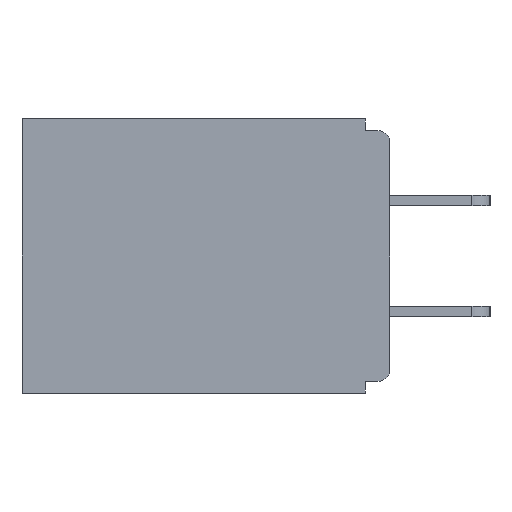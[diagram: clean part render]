
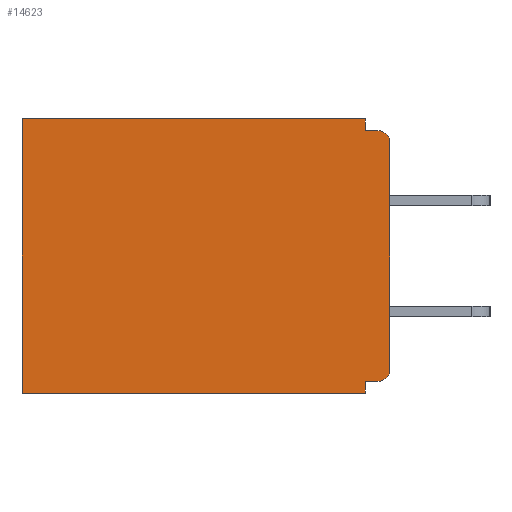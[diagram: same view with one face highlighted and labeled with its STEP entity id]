
A CAD part, left-side view. The second image highlights one B-rep face of the part: STEP entity #14623.
In plain terms, the highlighted planar face has unit normal (-1, 0, 0).
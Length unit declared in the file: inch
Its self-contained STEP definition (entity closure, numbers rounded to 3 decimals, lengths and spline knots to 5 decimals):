
#581 = CARTESIAN_POINT ( 'NONE',  ( 0.298, 0., -0.03 ) ) ;
#639 = CARTESIAN_POINT ( 'NONE',  ( 0.298, 0.46, 0. ) ) ;
#872 = VERTEX_POINT ( 'NONE', #6271 ) ;
#1793 = EDGE_CURVE ( 'NONE', #19414, #14546, #3138, .T. ) ;
#1974 = ORIENTED_EDGE ( 'NONE', *, *, #3672, .F. ) ;
#2142 = EDGE_CURVE ( 'NONE', #9829, #6226, #15710, .T. ) ;
#2200 = EDGE_CURVE ( 'NONE', #872, #7360, #11636, .T. ) ;
#2210 = CARTESIAN_POINT ( 'NONE',  ( 0.298, 0.46, -0.343 ) ) ;
#2600 = CARTESIAN_POINT ( 'NONE',  ( 0.298, 0.031, -0.343 ) ) ;
#2861 = CARTESIAN_POINT ( 'NONE',  ( 0.298, 0.015, -0.015 ) ) ;
#3009 = EDGE_CURVE ( 'NONE', #4221, #872, #5028, .T. ) ;
#3138 = LINE ( 'NONE', #11906, #14774 ) ;
#3296 = CARTESIAN_POINT ( 'NONE',  ( 0.298, 0.015, -0.328 ) ) ;
#3672 = EDGE_CURVE ( 'NONE', #4221, #16984, #13255, .T. ) ;
#4221 = VERTEX_POINT ( 'NONE', #19803 ) ;
#4634 = FACE_OUTER_BOUND ( 'NONE', #7765, .T. ) ;
#4674 = DIRECTION ( 'NONE',  ( -1., 0., 0. ) ) ;
#5028 = LINE ( 'NONE', #6264, #16907 ) ;
#5146 = CARTESIAN_POINT ( 'NONE',  ( 0.298, 0., -0.015 ) ) ;
#5211 = DIRECTION ( 'NONE',  ( 0., 0., -1. ) ) ;
#5227 = ORIENTED_EDGE ( 'NONE', *, *, #12411, .F. ) ;
#6051 = PLANE ( 'NONE',  #15280 ) ;
#6153 = VECTOR ( 'NONE', #16718, 39.37008 ) ;
#6226 = VERTEX_POINT ( 'NONE', #2861 ) ;
#6264 = CARTESIAN_POINT ( 'NONE',  ( 0.298, 0., 0. ) ) ;
#6271 = CARTESIAN_POINT ( 'NONE',  ( 0.298, 0.46, 0. ) ) ;
#6569 = CARTESIAN_POINT ( 'NONE',  ( 0.298, 0.031, -0.328 ) ) ;
#6832 = CIRCLE ( 'NONE', #8032, 0.015 ) ;
#7230 = DIRECTION ( 'NONE',  ( 0., 0., -1. ) ) ;
#7360 = VERTEX_POINT ( 'NONE', #2210 ) ;
#7461 = VECTOR ( 'NONE', #5211, 39.37008 ) ;
#7633 = CARTESIAN_POINT ( 'NONE',  ( 0.298, 0., 0. ) ) ;
#7765 = EDGE_LOOP ( 'NONE', ( #16292, #5227, #1974, #17564, #18570, #19208, #14163, #19830, #9957, #11069 ) ) ;
#8001 = EDGE_CURVE ( 'NONE', #19301, #19414, #15339, .T. ) ;
#8032 = AXIS2_PLACEMENT_3D ( 'NONE', #14561, #17488, #8374 ) ;
#8374 = DIRECTION ( 'NONE',  ( 0., 0., -1. ) ) ;
#8900 = VECTOR ( 'NONE', #11335, 39.37008 ) ;
#9829 = VERTEX_POINT ( 'NONE', #581 ) ;
#9905 = DIRECTION ( 'NONE',  ( 0., 0., -1. ) ) ;
#9957 = ORIENTED_EDGE ( 'NONE', *, *, #14473, .T. ) ;
#10480 = DIRECTION ( 'NONE',  ( 0., 0., -1. ) ) ;
#11069 = ORIENTED_EDGE ( 'NONE', *, *, #17675, .F. ) ;
#11266 = DIRECTION ( 'NONE',  ( 0., 1., 0. ) ) ;
#11335 = DIRECTION ( 'NONE',  ( 0., -1., 0. ) ) ;
#11636 = LINE ( 'NONE', #639, #19401 ) ;
#11683 = LINE ( 'NONE', #15967, #16257 ) ;
#11793 = LINE ( 'NONE', #14545, #7461 ) ;
#11906 = CARTESIAN_POINT ( 'NONE',  ( 0.298, 0.031, -0.343 ) ) ;
#12411 = EDGE_CURVE ( 'NONE', #16984, #6226, #14415, .T. ) ;
#12762 = VECTOR ( 'NONE', #15110, 39.37008 ) ;
#13255 = LINE ( 'NONE', #18117, #12762 ) ;
#14163 = ORIENTED_EDGE ( 'NONE', *, *, #1793, .F. ) ;
#14415 = LINE ( 'NONE', #5146, #8900 ) ;
#14426 = CARTESIAN_POINT ( 'NONE',  ( 0.298, 0.031, -0.015 ) ) ;
#14473 = EDGE_CURVE ( 'NONE', #19301, #18134, #6832, .T. ) ;
#14545 = CARTESIAN_POINT ( 'NONE',  ( 0.298, 0., 0. ) ) ;
#14546 = VERTEX_POINT ( 'NONE', #2600 ) ;
#14561 = CARTESIAN_POINT ( 'NONE',  ( 0.298, 0.015, -0.313 ) ) ;
#14623 = ADVANCED_FACE ( 'NONE', ( #4634 ), #6051, .F. ) ;
#14774 = VECTOR ( 'NONE', #7230, 39.37008 ) ;
#15110 = DIRECTION ( 'NONE',  ( 0., 0., -1. ) ) ;
#15172 = CARTESIAN_POINT ( 'NONE',  ( 0.298, 0., -0.328 ) ) ;
#15280 = AXIS2_PLACEMENT_3D ( 'NONE', #7633, #19822, #10480 ) ;
#15339 = LINE ( 'NONE', #15172, #6153 ) ;
#15710 = CIRCLE ( 'NONE', #19223, 0.015 ) ;
#15944 = CARTESIAN_POINT ( 'NONE',  ( 0.298, 0.015, -0.03 ) ) ;
#15967 = CARTESIAN_POINT ( 'NONE',  ( 0.298, 0., -0.343 ) ) ;
#16257 = VECTOR ( 'NONE', #11266, 39.37008 ) ;
#16292 = ORIENTED_EDGE ( 'NONE', *, *, #2142, .T. ) ;
#16718 = DIRECTION ( 'NONE',  ( 0., 1., 0. ) ) ;
#16907 = VECTOR ( 'NONE', #17078, 39.37008 ) ;
#16984 = VERTEX_POINT ( 'NONE', #14426 ) ;
#17078 = DIRECTION ( 'NONE',  ( 0., 1., 0. ) ) ;
#17379 = CARTESIAN_POINT ( 'NONE',  ( 0.298, 0., -0.313 ) ) ;
#17383 = DIRECTION ( 'NONE',  ( 0., 0., -1. ) ) ;
#17488 = DIRECTION ( 'NONE',  ( -1., 0., 0. ) ) ;
#17564 = ORIENTED_EDGE ( 'NONE', *, *, #3009, .T. ) ;
#17675 = EDGE_CURVE ( 'NONE', #9829, #18134, #11793, .T. ) ;
#18117 = CARTESIAN_POINT ( 'NONE',  ( 0.298, 0.031, -0.343 ) ) ;
#18134 = VERTEX_POINT ( 'NONE', #17379 ) ;
#18570 = ORIENTED_EDGE ( 'NONE', *, *, #2200, .T. ) ;
#19043 = EDGE_CURVE ( 'NONE', #14546, #7360, #11683, .T. ) ;
#19208 = ORIENTED_EDGE ( 'NONE', *, *, #19043, .F. ) ;
#19223 = AXIS2_PLACEMENT_3D ( 'NONE', #15944, #4674, #17383 ) ;
#19301 = VERTEX_POINT ( 'NONE', #3296 ) ;
#19401 = VECTOR ( 'NONE', #9905, 39.37008 ) ;
#19414 = VERTEX_POINT ( 'NONE', #6569 ) ;
#19803 = CARTESIAN_POINT ( 'NONE',  ( 0.298, 0.031, 0. ) ) ;
#19822 = DIRECTION ( 'NONE',  ( 1., 0., 0. ) ) ;
#19830 = ORIENTED_EDGE ( 'NONE', *, *, #8001, .F. ) ;
